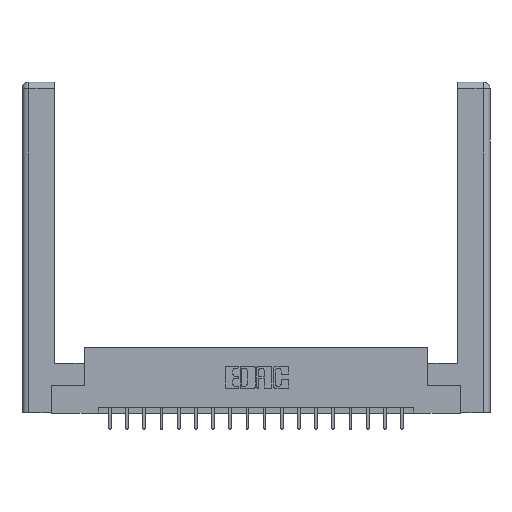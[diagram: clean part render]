
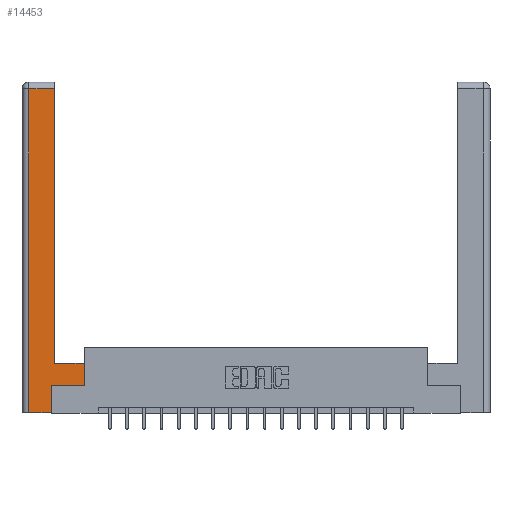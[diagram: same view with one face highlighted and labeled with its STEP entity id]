
A CAD part, top view. The second image highlights one B-rep face of the part: STEP entity #14453.
In plain terms, the highlighted planar face has unit normal (0, 0, 1).
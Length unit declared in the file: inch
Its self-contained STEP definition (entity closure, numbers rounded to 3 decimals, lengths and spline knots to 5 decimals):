
#1016 = CARTESIAN_POINT ( 'NONE',  ( 0.0615, 2.94, 0. ) ) ;
#1191 = VECTOR ( 'NONE', #6462, 39.37008 ) ;
#1332 = DIRECTION ( 'NONE',  ( 0., -1., 0. ) ) ;
#1421 = ORIENTED_EDGE ( 'NONE', *, *, #10465, .T. ) ;
#1929 = VERTEX_POINT ( 'NONE', #3548 ) ;
#2056 = CARTESIAN_POINT ( 'NONE',  ( 0.265, 0., 0. ) ) ;
#2057 = VECTOR ( 'NONE', #17262, 39.37008 ) ;
#2238 = LINE ( 'NONE', #6108, #15781 ) ;
#2389 = FACE_OUTER_BOUND ( 'NONE', #10266, .T. ) ;
#2807 = VERTEX_POINT ( 'NONE', #10428 ) ;
#2960 = LINE ( 'NONE', #4401, #18687 ) ;
#3139 = ORIENTED_EDGE ( 'NONE', *, *, #10885, .T. ) ;
#3448 = VECTOR ( 'NONE', #10347, 39.37008 ) ;
#3548 = CARTESIAN_POINT ( 'NONE',  ( 0.295, 0.45, 0. ) ) ;
#3856 = EDGE_CURVE ( 'NONE', #2807, #19263, #6757, .T. ) ;
#3909 = LINE ( 'NONE', #19591, #5090 ) ;
#3962 = ORIENTED_EDGE ( 'NONE', *, *, #9874, .T. ) ;
#4401 = CARTESIAN_POINT ( 'NONE',  ( 0.565, 0.245, 0. ) ) ;
#4475 = ORIENTED_EDGE ( 'NONE', *, *, #11697, .T. ) ;
#5090 = VECTOR ( 'NONE', #7441, 39.37008 ) ;
#5454 = DIRECTION ( 'NONE',  ( 0., 0., -1. ) ) ;
#5751 = DIRECTION ( 'NONE',  ( 0., 1., 0. ) ) ;
#5872 = DIRECTION ( 'NONE',  ( 1., 0., 0. ) ) ;
#6108 = CARTESIAN_POINT ( 'NONE',  ( 0.0615, 0., 0. ) ) ;
#6408 = CARTESIAN_POINT ( 'NONE',  ( 0.0615, 0., 0. ) ) ;
#6462 = DIRECTION ( 'NONE',  ( 0., 1., 0. ) ) ;
#6757 = LINE ( 'NONE', #10225, #3448 ) ;
#6787 = LINE ( 'NONE', #7875, #9875 ) ;
#6788 = CARTESIAN_POINT ( 'NONE',  ( 0., 0., 0. ) ) ;
#7441 = DIRECTION ( 'NONE',  ( 0., 1., 0. ) ) ;
#7875 = CARTESIAN_POINT ( 'NONE',  ( 0.265, 0., 0. ) ) ;
#8060 = AXIS2_PLACEMENT_3D ( 'NONE', #6788, #5454, #19053 ) ;
#8509 = EDGE_CURVE ( 'NONE', #8905, #16148, #10901, .T. ) ;
#8905 = VERTEX_POINT ( 'NONE', #16362 ) ;
#9702 = ORIENTED_EDGE ( 'NONE', *, *, #3856, .T. ) ;
#9874 = EDGE_CURVE ( 'NONE', #9939, #14270, #6787, .T. ) ;
#9875 = VECTOR ( 'NONE', #15574, 39.37008 ) ;
#9939 = VERTEX_POINT ( 'NONE', #6408 ) ;
#10024 = ORIENTED_EDGE ( 'NONE', *, *, #14450, .T. ) ;
#10225 = CARTESIAN_POINT ( 'NONE',  ( 0.0615, 2.94, 0. ) ) ;
#10266 = EDGE_LOOP ( 'NONE', ( #10024, #9702, #4475, #3962, #3139, #1421, #14244, #15424 ) ) ;
#10347 = DIRECTION ( 'NONE',  ( -1., 0., 0. ) ) ;
#10428 = CARTESIAN_POINT ( 'NONE',  ( 0.295, 2.94, 0. ) ) ;
#10465 = EDGE_CURVE ( 'NONE', #12391, #8905, #2960, .T. ) ;
#10885 = EDGE_CURVE ( 'NONE', #14270, #12391, #3909, .T. ) ;
#10901 = LINE ( 'NONE', #14681, #11853 ) ;
#11349 = CARTESIAN_POINT ( 'NONE',  ( 0.295, 0.45, 0. ) ) ;
#11697 = EDGE_CURVE ( 'NONE', #19263, #9939, #2238, .T. ) ;
#11853 = VECTOR ( 'NONE', #5751, 39.37008 ) ;
#12391 = VERTEX_POINT ( 'NONE', #14185 ) ;
#13870 = CARTESIAN_POINT ( 'NONE',  ( 0.565, 0.45, 0. ) ) ;
#14131 = CARTESIAN_POINT ( 'NONE',  ( 0.295, 3., 0. ) ) ;
#14185 = CARTESIAN_POINT ( 'NONE',  ( 0.265, 0.245, 0. ) ) ;
#14244 = ORIENTED_EDGE ( 'NONE', *, *, #8509, .T. ) ;
#14270 = VERTEX_POINT ( 'NONE', #2056 ) ;
#14450 = EDGE_CURVE ( 'NONE', #1929, #2807, #18568, .T. ) ;
#14453 = ADVANCED_FACE ( 'NONE', ( #2389 ), #15562, .F. ) ;
#14664 = LINE ( 'NONE', #11349, #2057 ) ;
#14681 = CARTESIAN_POINT ( 'NONE',  ( 0.565, 0.45, 0. ) ) ;
#15424 = ORIENTED_EDGE ( 'NONE', *, *, #16394, .T. ) ;
#15562 = PLANE ( 'NONE',  #8060 ) ;
#15574 = DIRECTION ( 'NONE',  ( 1., 0., 0. ) ) ;
#15781 = VECTOR ( 'NONE', #1332, 39.37008 ) ;
#16148 = VERTEX_POINT ( 'NONE', #13870 ) ;
#16362 = CARTESIAN_POINT ( 'NONE',  ( 0.565, 0.245, 0. ) ) ;
#16394 = EDGE_CURVE ( 'NONE', #16148, #1929, #14664, .T. ) ;
#17262 = DIRECTION ( 'NONE',  ( -1., 0., 0. ) ) ;
#18568 = LINE ( 'NONE', #14131, #1191 ) ;
#18687 = VECTOR ( 'NONE', #5872, 39.37008 ) ;
#19053 = DIRECTION ( 'NONE',  ( -1., 0., 0. ) ) ;
#19263 = VERTEX_POINT ( 'NONE', #1016 ) ;
#19591 = CARTESIAN_POINT ( 'NONE',  ( 0.265, 0.245, 0. ) ) ;
